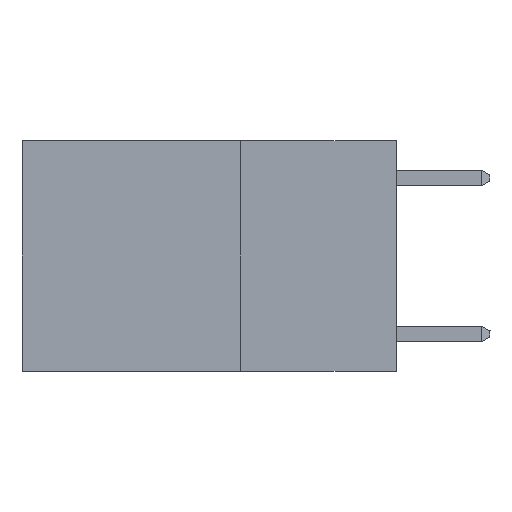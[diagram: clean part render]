
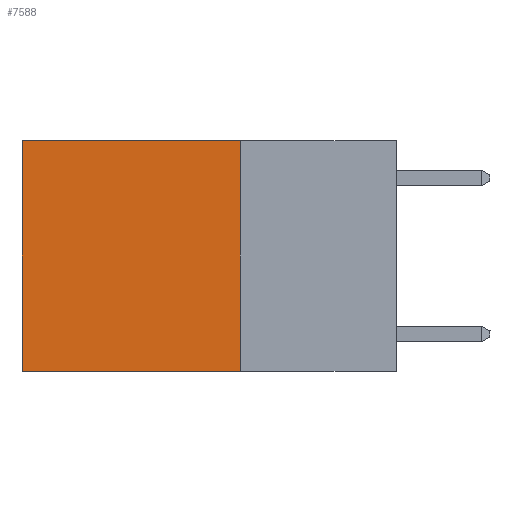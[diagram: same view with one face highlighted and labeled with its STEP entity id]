
A CAD part, left-side view. The second image highlights one B-rep face of the part: STEP entity #7588.
In plain terms, the highlighted planar face has unit normal (-1, 0, 0).
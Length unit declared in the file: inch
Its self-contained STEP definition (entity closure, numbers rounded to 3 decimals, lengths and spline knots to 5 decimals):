
#679 = CARTESIAN_POINT ( 'NONE',  ( 0.2625, 0.25, 0. ) ) ;
#1611 = VERTEX_POINT ( 'NONE', #2855 ) ;
#1893 = ORIENTED_EDGE ( 'NONE', *, *, #6071, .T. ) ;
#2136 = EDGE_CURVE ( 'NONE', #1611, #13890, #5874, .T. ) ;
#2600 = CARTESIAN_POINT ( 'NONE',  ( 0.2625, 0.25, 0. ) ) ;
#2739 = ORIENTED_EDGE ( 'NONE', *, *, #5494, .T. ) ;
#2757 = VERTEX_POINT ( 'NONE', #10537 ) ;
#2855 = CARTESIAN_POINT ( 'NONE',  ( 0.2625, 0.25, 0. ) ) ;
#3065 = AXIS2_PLACEMENT_3D ( 'NONE', #2600, #5658, #3645 ) ;
#3206 = ORIENTED_EDGE ( 'NONE', *, *, #2136, .F. ) ;
#3645 = DIRECTION ( 'NONE',  ( 0., 0., -1. ) ) ;
#3862 = CARTESIAN_POINT ( 'NONE',  ( 0.2625, 0.6, 0. ) ) ;
#4079 = LINE ( 'NONE', #679, #4581 ) ;
#4581 = VECTOR ( 'NONE', #7219, 39.37008 ) ;
#4954 = DIRECTION ( 'NONE',  ( 0., 0., -1. ) ) ;
#5231 = DIRECTION ( 'NONE',  ( 0., 0., -1. ) ) ;
#5494 = EDGE_CURVE ( 'NONE', #8198, #2757, #11399, .T. ) ;
#5658 = DIRECTION ( 'NONE',  ( 1., 0., 0. ) ) ;
#5874 = LINE ( 'NONE', #10572, #7426 ) ;
#6071 = EDGE_CURVE ( 'NONE', #1611, #8198, #4079, .T. ) ;
#6192 = DIRECTION ( 'NONE',  ( 0., 1., 0. ) ) ;
#7219 = DIRECTION ( 'NONE',  ( 0., 1., 0. ) ) ;
#7426 = VECTOR ( 'NONE', #5231, 39.37008 ) ;
#7588 = ADVANCED_FACE ( 'NONE', ( #8313 ), #12319, .F. ) ;
#7837 = VECTOR ( 'NONE', #4954, 39.37008 ) ;
#8198 = VERTEX_POINT ( 'NONE', #8325 ) ;
#8313 = FACE_OUTER_BOUND ( 'NONE', #11132, .T. ) ;
#8325 = CARTESIAN_POINT ( 'NONE',  ( 0.2625, 0.6, 0. ) ) ;
#9168 = EDGE_CURVE ( 'NONE', #13890, #2757, #12150, .T. ) ;
#9209 = CARTESIAN_POINT ( 'NONE',  ( 0.2625, 0.25, -0.37 ) ) ;
#10537 = CARTESIAN_POINT ( 'NONE',  ( 0.2625, 0.6, -0.37 ) ) ;
#10572 = CARTESIAN_POINT ( 'NONE',  ( 0.2625, 0.25, 0. ) ) ;
#10970 = VECTOR ( 'NONE', #6192, 39.37008 ) ;
#11132 = EDGE_LOOP ( 'NONE', ( #2739, #12162, #3206, #1893 ) ) ;
#11399 = LINE ( 'NONE', #3862, #7837 ) ;
#12150 = LINE ( 'NONE', #13657, #10970 ) ;
#12162 = ORIENTED_EDGE ( 'NONE', *, *, #9168, .F. ) ;
#12319 = PLANE ( 'NONE',  #3065 ) ;
#13657 = CARTESIAN_POINT ( 'NONE',  ( 0.2625, 0.25, -0.37 ) ) ;
#13890 = VERTEX_POINT ( 'NONE', #9209 ) ;
